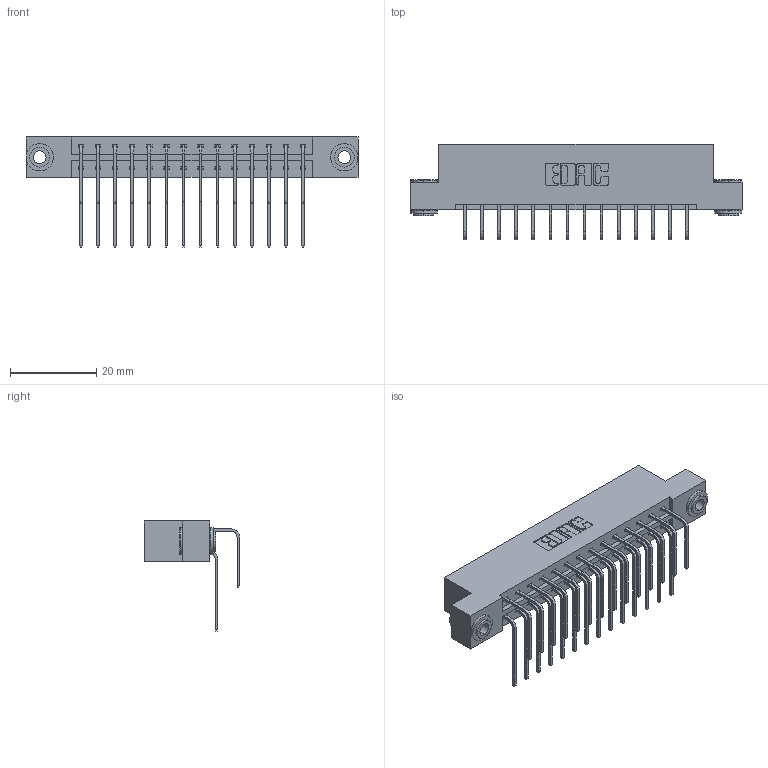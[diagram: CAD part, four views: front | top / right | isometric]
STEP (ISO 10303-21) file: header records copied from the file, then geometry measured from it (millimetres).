
FILE_DESCRIPTION (( 'STEP AP203' ), '1' );
FILE_NAME ('333-028-558-203.STEP', '2018-08-02T15:46:54', ( '' ), ( '' ), 'SwSTEP 2.0', 'SolidWorks 2016', '' );
FILE_SCHEMA (( 'CONFIG_CONTROL_DESIGN' ));
Length unit declared in the file: inch
Products named in the file (5): 345-292-001_558 Tail - 2; 345-250-002_345-250-002-102; 333-028-558-203; 333 Part_Flush - .156 Dia - TH; 345-292-001_558 559 Tail - 1
Assembly tree (31 placements, depth 2):
  333-028-558-203
    333 Part_Flush - .156 Dia - TH
    345-292-001_558 559 Tail - 1  x14
    345-292-001_558 Tail - 2  x14
    345-250-002_345-250-002-102  x2
Bounding box: 77.01 x 22.17 x 25.53 mm (x, y, z)
Volume: 7781.6 mm3; surface area: 9924.4 mm2
Topology: 31 solids, 31 shells, 1664 faces, 4895 edges, 3222 vertices
Faces by surface type: plane 1144, cylinder 512, cone 8
Entity records: 15062 total; most frequent: CARTESIAN_POINT 2556, ORIENTED_EDGE 2434, DIRECTION 2247, EDGE_CURVE 1217, VECTOR 1025, LINE 1025, VERTEX_POINT 806, AXIS2_PLACEMENT_3D 611
